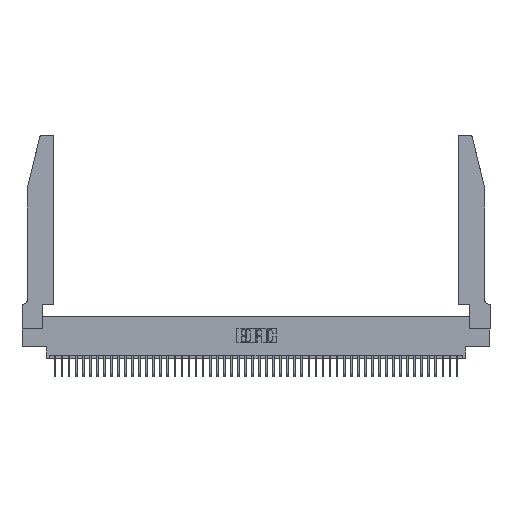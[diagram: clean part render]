
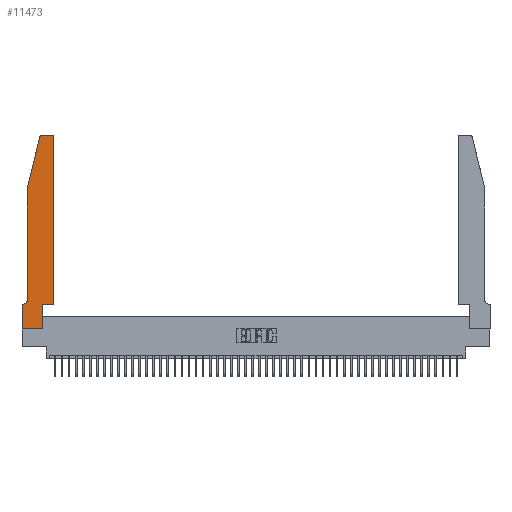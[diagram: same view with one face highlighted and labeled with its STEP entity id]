
A CAD part, top view. The second image highlights one B-rep face of the part: STEP entity #11473.
In plain terms, the highlighted planar face has unit normal (0, 0, 1).
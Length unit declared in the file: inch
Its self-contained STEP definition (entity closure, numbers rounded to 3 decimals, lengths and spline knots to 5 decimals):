
#1160 = AXIS2_PLACEMENT_3D ( 'NONE', #5748, #21451, #21789 ) ;
#1508 = VERTEX_POINT ( 'NONE', #45689 ) ;
#1864 = VECTOR ( 'NONE', #26537, 39.37008 ) ;
#2039 = DIRECTION ( 'NONE',  ( 0., -1., 0. ) ) ;
#2196 = VECTOR ( 'NONE', #20082, 39.37008 ) ;
#2520 = DIRECTION ( 'NONE',  ( 0., 0., 1. ) ) ;
#3873 = CARTESIAN_POINT ( 'NONE',  ( 0., 0., 0.37 ) ) ;
#5048 = VERTEX_POINT ( 'NONE', #6143 ) ;
#5748 = CARTESIAN_POINT ( 'NONE',  ( 0.284, 2.72, 0.37 ) ) ;
#6143 = CARTESIAN_POINT ( 'NONE',  ( 0., 0.35, 0.37 ) ) ;
#6383 = DIRECTION ( 'NONE',  ( 1., 0., 0. ) ) ;
#6459 = AXIS2_PLACEMENT_3D ( 'NONE', #21780, #2520, #6383 ) ;
#6713 = VERTEX_POINT ( 'NONE', #11338 ) ;
#7191 = AXIS2_PLACEMENT_3D ( 'NONE', #24247, #16301, #23914 ) ;
#7454 = EDGE_CURVE ( 'NONE', #6713, #32429, #39415, .T. ) ;
#7861 = LINE ( 'NONE', #19762, #33185 ) ;
#8051 = CARTESIAN_POINT ( 'NONE',  ( 0.0755, 0.35, 0.37 ) ) ;
#8534 = CARTESIAN_POINT ( 'NONE',  ( 0.284, 2.75, 0.37 ) ) ;
#8942 = VECTOR ( 'NONE', #11712, 39.37008 ) ;
#9383 = VERTEX_POINT ( 'NONE', #45255 ) ;
#9483 = ORIENTED_EDGE ( 'NONE', *, *, #17103, .T. ) ;
#9875 = VECTOR ( 'NONE', #33475, 39.37008 ) ;
#10620 = VERTEX_POINT ( 'NONE', #3873 ) ;
#10629 = ORIENTED_EDGE ( 'NONE', *, *, #36545, .T. ) ;
#10746 = VECTOR ( 'NONE', #28849, 39.37008 ) ;
#11011 = ORIENTED_EDGE ( 'NONE', *, *, #24890, .T. ) ;
#11338 = CARTESIAN_POINT ( 'NONE',  ( 0.4205, 2.75, 0.37 ) ) ;
#11473 = ADVANCED_FACE ( 'NONE', ( #44484 ), #32353, .T. ) ;
#11712 = DIRECTION ( 'NONE',  ( 0., 1., 0. ) ) ;
#11944 = EDGE_CURVE ( 'NONE', #37269, #32130, #27957, .T. ) ;
#12249 = VECTOR ( 'NONE', #46763, 39.37008 ) ;
#13226 = CARTESIAN_POINT ( 'NONE',  ( 0.4505, 2.72, 0.37 ) ) ;
#14429 = LINE ( 'NONE', #16764, #10746 ) ;
#15300 = EDGE_CURVE ( 'NONE', #5048, #10620, #14429, .T. ) ;
#15434 = VERTEX_POINT ( 'NONE', #21937 ) ;
#15928 = ORIENTED_EDGE ( 'NONE', *, *, #15300, .T. ) ;
#15966 = CARTESIAN_POINT ( 'NONE',  ( 0.25487, 2.72718, 0.37 ) ) ;
#16301 = DIRECTION ( 'NONE',  ( 0., 0., -1. ) ) ;
#16565 = VECTOR ( 'NONE', #48575, 39.37008 ) ;
#16746 = LINE ( 'NONE', #8051, #2196 ) ;
#16764 = CARTESIAN_POINT ( 'NONE',  ( 0., 0., 0.37 ) ) ;
#17044 = DIRECTION ( 'NONE',  ( 0., 0., 1. ) ) ;
#17103 = EDGE_CURVE ( 'NONE', #9383, #37269, #45551, .T. ) ;
#19689 = CARTESIAN_POINT ( 'NONE',  ( 0.2605, 2.75, 0.37 ) ) ;
#19762 = CARTESIAN_POINT ( 'NONE',  ( 0.4505, 0.35, 0.37 ) ) ;
#19995 = VERTEX_POINT ( 'NONE', #42516 ) ;
#20082 = DIRECTION ( 'NONE',  ( -1., 0., 0. ) ) ;
#21409 = VERTEX_POINT ( 'NONE', #15966 ) ;
#21415 = ORIENTED_EDGE ( 'NONE', *, *, #11944, .T. ) ;
#21451 = DIRECTION ( 'NONE',  ( 0., 0., 1. ) ) ;
#21552 = CARTESIAN_POINT ( 'NONE',  ( 0.0755, 0.42, 0.37 ) ) ;
#21780 = CARTESIAN_POINT ( 'NONE',  ( 0.4205, 2.72, 0.37 ) ) ;
#21789 = DIRECTION ( 'NONE',  ( 1., 0., 0. ) ) ;
#21937 = CARTESIAN_POINT ( 'NONE',  ( 0.4505, 0.35, 0.37 ) ) ;
#22360 = CIRCLE ( 'NONE', #1160, 0.03 ) ;
#23914 = DIRECTION ( 'NONE',  ( -1., 0., 0. ) ) ;
#24247 = CARTESIAN_POINT ( 'NONE',  ( 0.0055, 0.42, 0.37 ) ) ;
#24793 = ORIENTED_EDGE ( 'NONE', *, *, #48300, .T. ) ;
#24890 = EDGE_CURVE ( 'NONE', #21409, #9383, #47295, .T. ) ;
#26287 = VECTOR ( 'NONE', #2039, 39.37008 ) ;
#26537 = DIRECTION ( 'NONE',  ( 1., 0., 0. ) ) ;
#26624 = ORIENTED_EDGE ( 'NONE', *, *, #7454, .T. ) ;
#27182 = CIRCLE ( 'NONE', #6459, 0.03 ) ;
#27786 = EDGE_LOOP ( 'NONE', ( #26624, #45692, #11011, #9483, #21415, #24793, #15928, #34689, #48175, #42041, #37747, #10629 ) ) ;
#27957 = CIRCLE ( 'NONE', #7191, 0.07 ) ;
#28389 = CARTESIAN_POINT ( 'NONE',  ( 0.0755, 2., 0.37 ) ) ;
#28448 = LINE ( 'NONE', #38464, #1864 ) ;
#28849 = DIRECTION ( 'NONE',  ( 0., -1., 0. ) ) ;
#29425 = LINE ( 'NONE', #35276, #8942 ) ;
#29587 = CARTESIAN_POINT ( 'NONE',  ( 0.2865, 0.35, 0.37 ) ) ;
#31651 = LINE ( 'NONE', #29587, #9875 ) ;
#32130 = VERTEX_POINT ( 'NONE', #33690 ) ;
#32353 = PLANE ( 'NONE',  #41754 ) ;
#32429 = VERTEX_POINT ( 'NONE', #8534 ) ;
#33185 = VECTOR ( 'NONE', #46679, 39.37008 ) ;
#33436 = CARTESIAN_POINT ( 'NONE',  ( 0.0755, 2., 0.37 ) ) ;
#33475 = DIRECTION ( 'NONE',  ( 0., 1., 0. ) ) ;
#33690 = CARTESIAN_POINT ( 'NONE',  ( 0.0055, 0.35, 0.37 ) ) ;
#34689 = ORIENTED_EDGE ( 'NONE', *, *, #36115, .T. ) ;
#35276 = CARTESIAN_POINT ( 'NONE',  ( 0.4505, 0.35, 0.37 ) ) ;
#36115 = EDGE_CURVE ( 'NONE', #10620, #19995, #28448, .T. ) ;
#36218 = CARTESIAN_POINT ( 'NONE',  ( 0., 0.35, 0.37 ) ) ;
#36545 = EDGE_CURVE ( 'NONE', #49186, #6713, #27182, .T. ) ;
#37269 = VERTEX_POINT ( 'NONE', #21552 ) ;
#37747 = ORIENTED_EDGE ( 'NONE', *, *, #38667, .T. ) ;
#38464 = CARTESIAN_POINT ( 'NONE',  ( 0., 0., 0.37 ) ) ;
#38667 = EDGE_CURVE ( 'NONE', #15434, #49186, #29425, .T. ) ;
#39415 = LINE ( 'NONE', #19689, #12249 ) ;
#40928 = EDGE_CURVE ( 'NONE', #19995, #1508, #31651, .T. ) ;
#41754 = AXIS2_PLACEMENT_3D ( 'NONE', #36218, #17044, #43958 ) ;
#42041 = ORIENTED_EDGE ( 'NONE', *, *, #43558, .T. ) ;
#42516 = CARTESIAN_POINT ( 'NONE',  ( 0.2865, 0., 0.37 ) ) ;
#43260 = EDGE_CURVE ( 'NONE', #32429, #21409, #22360, .T. ) ;
#43558 = EDGE_CURVE ( 'NONE', #1508, #15434, #7861, .T. ) ;
#43958 = DIRECTION ( 'NONE',  ( 1., 0., 0. ) ) ;
#44484 = FACE_OUTER_BOUND ( 'NONE', #27786, .T. ) ;
#45255 = CARTESIAN_POINT ( 'NONE',  ( 0.0755, 2., 0.37 ) ) ;
#45551 = LINE ( 'NONE', #33436, #26287 ) ;
#45689 = CARTESIAN_POINT ( 'NONE',  ( 0.2865, 0.35, 0.37 ) ) ;
#45692 = ORIENTED_EDGE ( 'NONE', *, *, #43260, .T. ) ;
#46679 = DIRECTION ( 'NONE',  ( 1., 0., 0. ) ) ;
#46763 = DIRECTION ( 'NONE',  ( -1., 0., 0. ) ) ;
#47295 = LINE ( 'NONE', #28389, #16565 ) ;
#48175 = ORIENTED_EDGE ( 'NONE', *, *, #40928, .T. ) ;
#48300 = EDGE_CURVE ( 'NONE', #32130, #5048, #16746, .T. ) ;
#48575 = DIRECTION ( 'NONE',  ( -0.239, -0.971, 0. ) ) ;
#49186 = VERTEX_POINT ( 'NONE', #13226 ) ;
